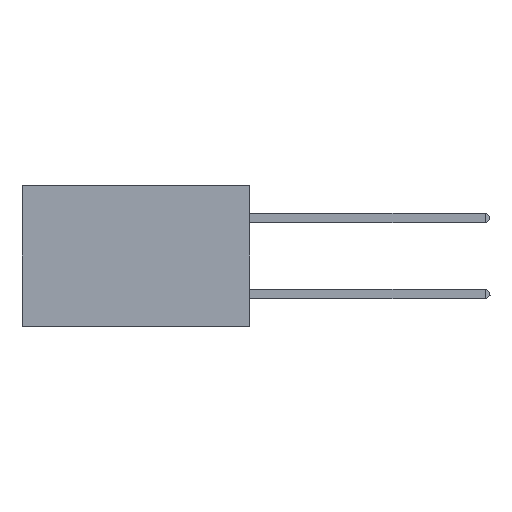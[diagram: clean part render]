
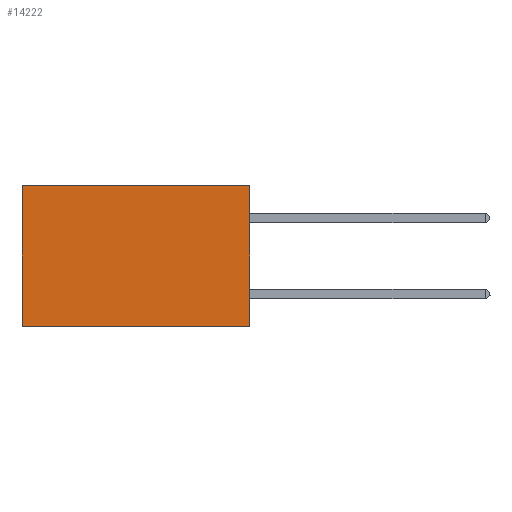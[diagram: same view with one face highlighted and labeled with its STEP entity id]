
A CAD part, left-side view. The second image highlights one B-rep face of the part: STEP entity #14222.
In plain terms, the highlighted planar face has unit normal (-1, 0, 0).
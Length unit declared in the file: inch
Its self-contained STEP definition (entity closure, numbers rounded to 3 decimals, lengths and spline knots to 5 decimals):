
#115 = CARTESIAN_POINT ( 'NONE',  ( 0.2875, 0., 0. ) ) ;
#713 = VECTOR ( 'NONE', #9512, 39.37008 ) ;
#1417 = LINE ( 'NONE', #115, #22323 ) ;
#2080 = EDGE_CURVE ( 'NONE', #8121, #3775, #24661, .T. ) ;
#2373 = CARTESIAN_POINT ( 'NONE',  ( 0.2875, 0.6, 0. ) ) ;
#2678 = CARTESIAN_POINT ( 'NONE',  ( 0.2875, 0., 0. ) ) ;
#3775 = VERTEX_POINT ( 'NONE', #4464 ) ;
#4328 = EDGE_CURVE ( 'NONE', #8121, #19211, #1417, .T. ) ;
#4464 = CARTESIAN_POINT ( 'NONE',  ( 0.2875, 0., -0.37 ) ) ;
#4704 = LINE ( 'NONE', #2373, #9161 ) ;
#6194 = VERTEX_POINT ( 'NONE', #13922 ) ;
#8121 = VERTEX_POINT ( 'NONE', #19611 ) ;
#9161 = VECTOR ( 'NONE', #18481, 39.37008 ) ;
#9512 = DIRECTION ( 'NONE',  ( 0., 1., 0. ) ) ;
#9601 = CARTESIAN_POINT ( 'NONE',  ( 0.2875, 0., -0.37 ) ) ;
#10548 = AXIS2_PLACEMENT_3D ( 'NONE', #2678, #16606, #22956 ) ;
#13084 = CARTESIAN_POINT ( 'NONE',  ( 0.2875, 0.6, 0. ) ) ;
#13234 = ORIENTED_EDGE ( 'NONE', *, *, #13911, .F. ) ;
#13911 = EDGE_CURVE ( 'NONE', #3775, #6194, #14044, .T. ) ;
#13922 = CARTESIAN_POINT ( 'NONE',  ( 0.2875, 0.6, -0.37 ) ) ;
#14044 = LINE ( 'NONE', #9601, #713 ) ;
#14157 = DIRECTION ( 'NONE',  ( 0., 0., -1. ) ) ;
#14222 = ADVANCED_FACE ( 'NONE', ( #18430 ), #22794, .F. ) ;
#14239 = CARTESIAN_POINT ( 'NONE',  ( 0.2875, 0., 0. ) ) ;
#15160 = ORIENTED_EDGE ( 'NONE', *, *, #17184, .T. ) ;
#16304 = ORIENTED_EDGE ( 'NONE', *, *, #2080, .F. ) ;
#16606 = DIRECTION ( 'NONE',  ( 1., 0., 0. ) ) ;
#17184 = EDGE_CURVE ( 'NONE', #19211, #6194, #4704, .T. ) ;
#17759 = EDGE_LOOP ( 'NONE', ( #15160, #13234, #16304, #23190 ) ) ;
#18430 = FACE_OUTER_BOUND ( 'NONE', #17759, .T. ) ;
#18481 = DIRECTION ( 'NONE',  ( 0., 0., -1. ) ) ;
#18614 = VECTOR ( 'NONE', #14157, 39.37008 ) ;
#19211 = VERTEX_POINT ( 'NONE', #13084 ) ;
#19611 = CARTESIAN_POINT ( 'NONE',  ( 0.2875, 0., 0. ) ) ;
#22323 = VECTOR ( 'NONE', #24718, 39.37008 ) ;
#22794 = PLANE ( 'NONE',  #10548 ) ;
#22956 = DIRECTION ( 'NONE',  ( 0., 0., -1. ) ) ;
#23190 = ORIENTED_EDGE ( 'NONE', *, *, #4328, .T. ) ;
#24661 = LINE ( 'NONE', #14239, #18614 ) ;
#24718 = DIRECTION ( 'NONE',  ( 0., 1., 0. ) ) ;
